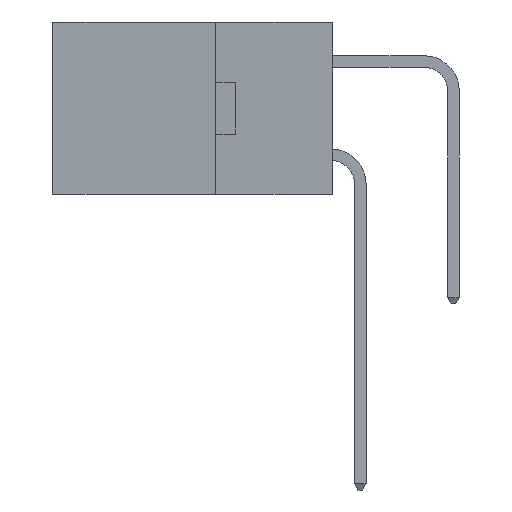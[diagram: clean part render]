
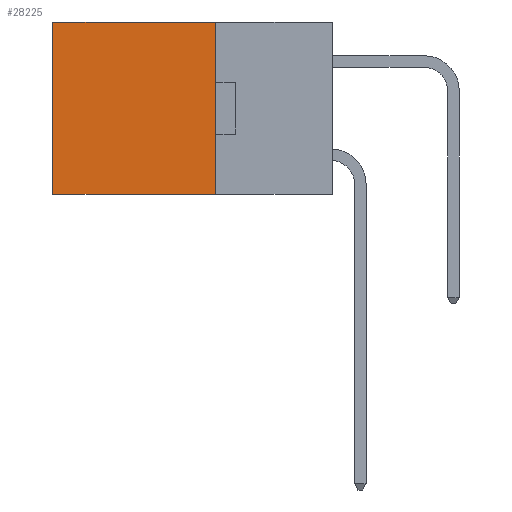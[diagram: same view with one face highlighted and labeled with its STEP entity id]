
A CAD part, left-side view. The second image highlights one B-rep face of the part: STEP entity #28225.
In plain terms, the highlighted planar face has unit normal (-1, 0, 0).
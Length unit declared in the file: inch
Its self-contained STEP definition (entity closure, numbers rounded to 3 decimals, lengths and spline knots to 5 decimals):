
#1594 = VERTEX_POINT ( 'NONE', #20390 ) ;
#1871 = ORIENTED_EDGE ( 'NONE', *, *, #6015, .T. ) ;
#3031 = DIRECTION ( 'NONE',  ( 1., 0., 0. ) ) ;
#3102 = LINE ( 'NONE', #18879, #14014 ) ;
#3285 = FACE_OUTER_BOUND ( 'NONE', #20441, .T. ) ;
#6015 = EDGE_CURVE ( 'NONE', #11341, #25057, #20323, .T. ) ;
#6310 = VECTOR ( 'NONE', #27905, 39.37008 ) ;
#6870 = CARTESIAN_POINT ( 'NONE',  ( 0.2615, 0.6, -0.37 ) ) ;
#6895 = EDGE_CURVE ( 'NONE', #1594, #9983, #12088, .T. ) ;
#8159 = AXIS2_PLACEMENT_3D ( 'NONE', #16065, #3031, #18289 ) ;
#9377 = VECTOR ( 'NONE', #23565, 39.37008 ) ;
#9842 = ORIENTED_EDGE ( 'NONE', *, *, #10119, .T. ) ;
#9983 = VERTEX_POINT ( 'NONE', #11397 ) ;
#10119 = EDGE_CURVE ( 'NONE', #1594, #11341, #17459, .T. ) ;
#11341 = VERTEX_POINT ( 'NONE', #16214 ) ;
#11397 = CARTESIAN_POINT ( 'NONE',  ( 0.2615, 0.25, -0.37 ) ) ;
#11869 = CARTESIAN_POINT ( 'NONE',  ( 0.2615, 0.25, 0. ) ) ;
#12088 = LINE ( 'NONE', #17035, #6310 ) ;
#12950 = ORIENTED_EDGE ( 'NONE', *, *, #6895, .F. ) ;
#14014 = VECTOR ( 'NONE', #18780, 39.37008 ) ;
#16065 = CARTESIAN_POINT ( 'NONE',  ( 0.2615, 0.25, -0.37 ) ) ;
#16214 = CARTESIAN_POINT ( 'NONE',  ( 0.2615, 0.6, 0. ) ) ;
#17035 = CARTESIAN_POINT ( 'NONE',  ( 0.2615, 0.25, -0.37 ) ) ;
#17459 = LINE ( 'NONE', #11869, #22584 ) ;
#18289 = DIRECTION ( 'NONE',  ( 0., 0., -1. ) ) ;
#18780 = DIRECTION ( 'NONE',  ( 0., 1., 0. ) ) ;
#18879 = CARTESIAN_POINT ( 'NONE',  ( 0.2615, 0.25, -0.37 ) ) ;
#18973 = EDGE_CURVE ( 'NONE', #9983, #25057, #3102, .T. ) ;
#20323 = LINE ( 'NONE', #21388, #9377 ) ;
#20390 = CARTESIAN_POINT ( 'NONE',  ( 0.2615, 0.25, 0. ) ) ;
#20441 = EDGE_LOOP ( 'NONE', ( #1871, #26702, #12950, #9842 ) ) ;
#21388 = CARTESIAN_POINT ( 'NONE',  ( 0.2615, 0.6, -0.37 ) ) ;
#22584 = VECTOR ( 'NONE', #22755, 39.37008 ) ;
#22755 = DIRECTION ( 'NONE',  ( 0., 1., 0. ) ) ;
#23565 = DIRECTION ( 'NONE',  ( 0., 0., -1. ) ) ;
#25057 = VERTEX_POINT ( 'NONE', #6870 ) ;
#26702 = ORIENTED_EDGE ( 'NONE', *, *, #18973, .F. ) ;
#26940 = PLANE ( 'NONE',  #8159 ) ;
#27905 = DIRECTION ( 'NONE',  ( 0., 0., -1. ) ) ;
#28225 = ADVANCED_FACE ( 'NONE', ( #3285 ), #26940, .F. ) ;
